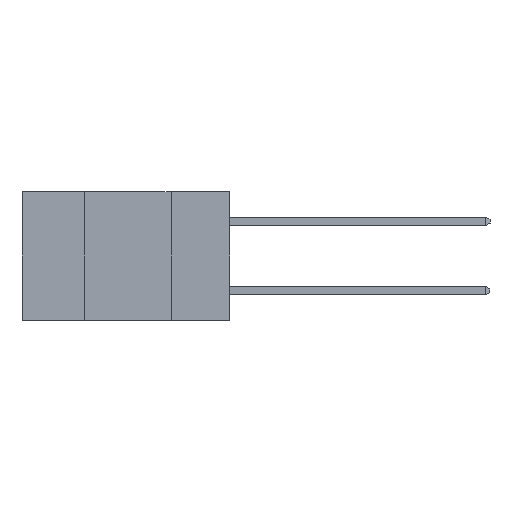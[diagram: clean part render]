
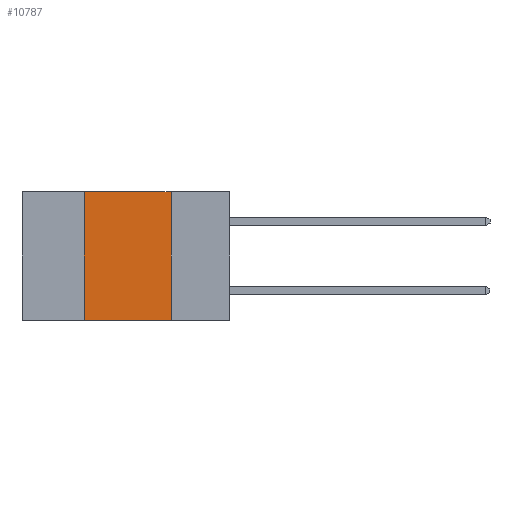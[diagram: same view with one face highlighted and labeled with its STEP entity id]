
A CAD part, left-side view. The second image highlights one B-rep face of the part: STEP entity #10787.
In plain terms, the highlighted planar face has unit normal (-1, 0, 0).
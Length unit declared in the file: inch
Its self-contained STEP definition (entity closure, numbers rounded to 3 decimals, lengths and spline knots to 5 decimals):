
#628 = FACE_OUTER_BOUND ( 'NONE', #7873, .T. ) ;
#3213 = LINE ( 'NONE', #12446, #9268 ) ;
#3269 = PLANE ( 'NONE',  #5243 ) ;
#3319 = DIRECTION ( 'NONE',  ( 0., 0., 1. ) ) ;
#3529 = EDGE_CURVE ( 'NONE', #9581, #6485, #14873, .T. ) ;
#3892 = ORIENTED_EDGE ( 'NONE', *, *, #7782, .F. ) ;
#4292 = ORIENTED_EDGE ( 'NONE', *, *, #3529, .F. ) ;
#4395 = DIRECTION ( 'NONE',  ( 0., -1., 0. ) ) ;
#4575 = DIRECTION ( 'NONE',  ( 0., 0., -1. ) ) ;
#4893 = EDGE_CURVE ( 'NONE', #6485, #13751, #5245, .T. ) ;
#5108 = CARTESIAN_POINT ( 'NONE',  ( 0., 0.42, 0. ) ) ;
#5243 = AXIS2_PLACEMENT_3D ( 'NONE', #5692, #11746, #4575 ) ;
#5245 = LINE ( 'NONE', #13401, #8044 ) ;
#5299 = VERTEX_POINT ( 'NONE', #7338 ) ;
#5692 = CARTESIAN_POINT ( 'NONE',  ( 0., 0.6, 0. ) ) ;
#6215 = CARTESIAN_POINT ( 'NONE',  ( 0., 0.6, -0.37 ) ) ;
#6299 = EDGE_CURVE ( 'NONE', #9581, #5299, #12377, .T. ) ;
#6485 = VERTEX_POINT ( 'NONE', #5108 ) ;
#6822 = DIRECTION ( 'NONE',  ( 0., -1., 0. ) ) ;
#7338 = CARTESIAN_POINT ( 'NONE',  ( 0., 0.17, -0.37 ) ) ;
#7782 = EDGE_CURVE ( 'NONE', #13751, #5299, #3213, .T. ) ;
#7873 = EDGE_LOOP ( 'NONE', ( #3892, #10268, #4292, #10654 ) ) ;
#8044 = VECTOR ( 'NONE', #6822, 39.37008 ) ;
#9268 = VECTOR ( 'NONE', #12610, 39.37008 ) ;
#9581 = VERTEX_POINT ( 'NONE', #15149 ) ;
#10268 = ORIENTED_EDGE ( 'NONE', *, *, #4893, .F. ) ;
#10654 = ORIENTED_EDGE ( 'NONE', *, *, #6299, .T. ) ;
#10787 = ADVANCED_FACE ( 'NONE', ( #628 ), #3269, .F. ) ;
#11746 = DIRECTION ( 'NONE',  ( 1., 0., 0. ) ) ;
#12377 = LINE ( 'NONE', #6215, #15186 ) ;
#12446 = CARTESIAN_POINT ( 'NONE',  ( 0., 0.17, 0. ) ) ;
#12610 = DIRECTION ( 'NONE',  ( 0., 0., -1. ) ) ;
#13401 = CARTESIAN_POINT ( 'NONE',  ( 0., 0.6, 0. ) ) ;
#13751 = VERTEX_POINT ( 'NONE', #14824 ) ;
#14495 = VECTOR ( 'NONE', #3319, 39.37008 ) ;
#14824 = CARTESIAN_POINT ( 'NONE',  ( 0., 0.17, 0. ) ) ;
#14873 = LINE ( 'NONE', #15105, #14495 ) ;
#15105 = CARTESIAN_POINT ( 'NONE',  ( 0., 0.42, 0. ) ) ;
#15149 = CARTESIAN_POINT ( 'NONE',  ( 0., 0.42, -0.37 ) ) ;
#15186 = VECTOR ( 'NONE', #4395, 39.37008 ) ;
